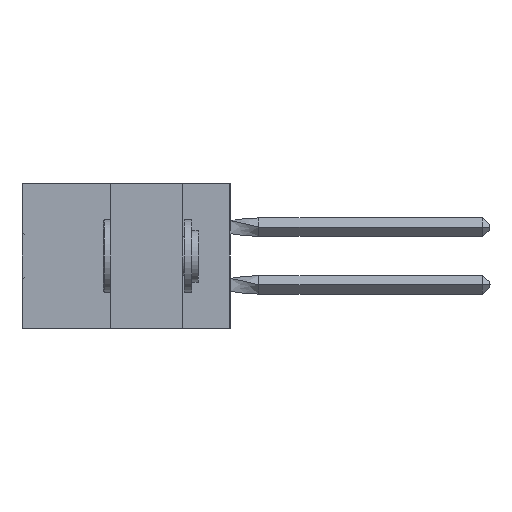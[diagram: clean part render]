
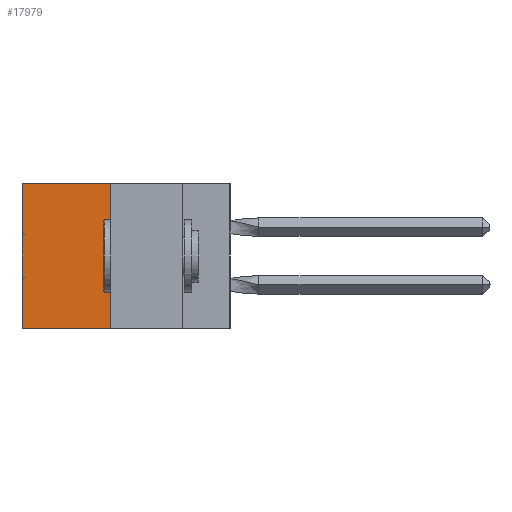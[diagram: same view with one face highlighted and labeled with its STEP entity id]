
A CAD part, left-side view. The second image highlights one B-rep face of the part: STEP entity #17979.
In plain terms, the highlighted planar face has unit normal (-1, 0, 0).
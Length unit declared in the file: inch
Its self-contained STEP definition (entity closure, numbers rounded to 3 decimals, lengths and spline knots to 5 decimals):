
#1861 = LINE ( 'NONE', #20024, #54116 ) ;
#1866 = VECTOR ( 'NONE', #6557, 39.37008 ) ;
#3440 = CARTESIAN_POINT ( 'NONE',  ( 0.305, 0.413, -0.5 ) ) ;
#3722 = EDGE_CURVE ( 'NONE', #36587, #19535, #46172, .T. ) ;
#4675 = FACE_OUTER_BOUND ( 'NONE', #51901, .T. ) ;
#6557 = DIRECTION ( 'NONE',  ( 0., 1., 0. ) ) ;
#8534 = LINE ( 'NONE', #43248, #38250 ) ;
#9563 = EDGE_CURVE ( 'NONE', #32451, #36587, #8534, .T. ) ;
#9888 = DIRECTION ( 'NONE',  ( 1., 0., 0. ) ) ;
#14509 = DIRECTION ( 'NONE',  ( 0., 0., -1. ) ) ;
#14922 = CARTESIAN_POINT ( 'NONE',  ( 0.305, 0.413, 0. ) ) ;
#15426 = DIRECTION ( 'NONE',  ( 0., 1., 0. ) ) ;
#16447 = VERTEX_POINT ( 'NONE', #28124 ) ;
#17926 = ORIENTED_EDGE ( 'NONE', *, *, #43882, .T. ) ;
#17979 = ADVANCED_FACE ( 'NONE', ( #4675 ), #51894, .F. ) ;
#18192 = CARTESIAN_POINT ( 'NONE',  ( 0.305, 0.413, -0.5 ) ) ;
#19434 = ORIENTED_EDGE ( 'NONE', *, *, #23467, .T. ) ;
#19535 = VERTEX_POINT ( 'NONE', #39433 ) ;
#20024 = CARTESIAN_POINT ( 'NONE',  ( 0.305, 0.413, 0. ) ) ;
#23467 = EDGE_CURVE ( 'NONE', #32451, #16447, #1861, .T. ) ;
#26968 = DIRECTION ( 'NONE',  ( 0., 0., -1. ) ) ;
#28124 = CARTESIAN_POINT ( 'NONE',  ( 0.305, 0.72, 0. ) ) ;
#30858 = LINE ( 'NONE', #41274, #42126 ) ;
#32451 = VERTEX_POINT ( 'NONE', #14922 ) ;
#35556 = CARTESIAN_POINT ( 'NONE',  ( 0.305, 0.413, -0.5 ) ) ;
#36587 = VERTEX_POINT ( 'NONE', #3440 ) ;
#38250 = VECTOR ( 'NONE', #26968, 39.37008 ) ;
#39433 = CARTESIAN_POINT ( 'NONE',  ( 0.305, 0.72, -0.5 ) ) ;
#41274 = CARTESIAN_POINT ( 'NONE',  ( 0.305, 0.72, -0.5 ) ) ;
#42126 = VECTOR ( 'NONE', #45534, 39.37008 ) ;
#42532 = ORIENTED_EDGE ( 'NONE', *, *, #9563, .F. ) ;
#43248 = CARTESIAN_POINT ( 'NONE',  ( 0.305, 0.413, -0.5 ) ) ;
#43882 = EDGE_CURVE ( 'NONE', #16447, #19535, #30858, .T. ) ;
#45289 = ORIENTED_EDGE ( 'NONE', *, *, #3722, .F. ) ;
#45534 = DIRECTION ( 'NONE',  ( 0., 0., -1. ) ) ;
#46172 = LINE ( 'NONE', #35556, #1866 ) ;
#47275 = AXIS2_PLACEMENT_3D ( 'NONE', #18192, #9888, #14509 ) ;
#51894 = PLANE ( 'NONE',  #47275 ) ;
#51901 = EDGE_LOOP ( 'NONE', ( #17926, #45289, #42532, #19434 ) ) ;
#54116 = VECTOR ( 'NONE', #15426, 39.37008 ) ;
